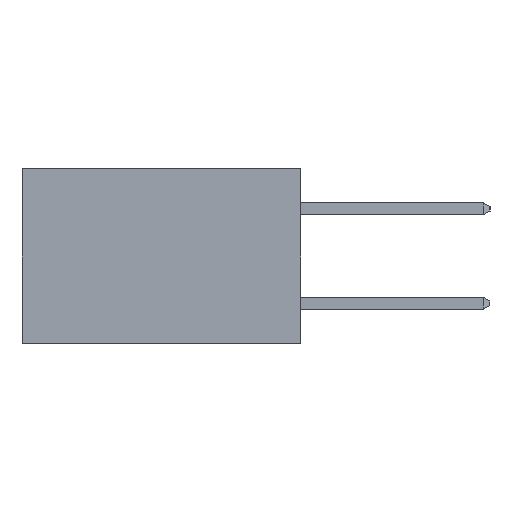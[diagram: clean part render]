
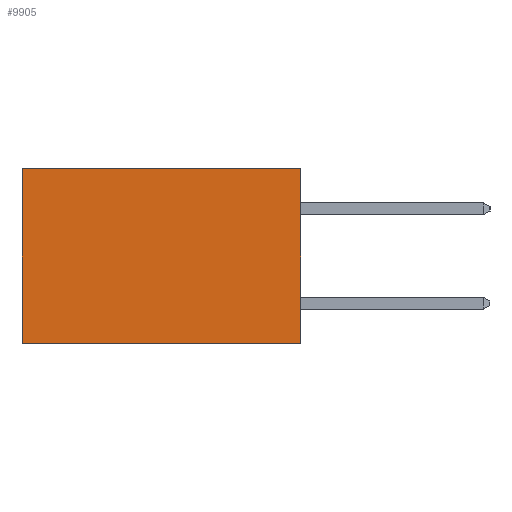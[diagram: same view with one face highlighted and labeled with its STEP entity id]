
A CAD part, left-side view. The second image highlights one B-rep face of the part: STEP entity #9905.
In plain terms, the highlighted planar face has unit normal (-1, 0, 0).
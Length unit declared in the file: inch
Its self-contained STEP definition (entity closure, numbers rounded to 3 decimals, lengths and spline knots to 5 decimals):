
#492 = VECTOR ( 'NONE', #8987, 39.37008 ) ;
#908 = LINE ( 'NONE', #6374, #19864 ) ;
#936 = CARTESIAN_POINT ( 'NONE',  ( 0.277, 0., 0. ) ) ;
#1145 = VERTEX_POINT ( 'NONE', #19620 ) ;
#2804 = DIRECTION ( 'NONE',  ( 1., 0., 0. ) ) ;
#3018 = CARTESIAN_POINT ( 'NONE',  ( 0.277, 0., -0.37 ) ) ;
#3370 = PLANE ( 'NONE',  #23247 ) ;
#4518 = CARTESIAN_POINT ( 'NONE',  ( 0.277, 0., -0.37 ) ) ;
#4908 = EDGE_CURVE ( 'NONE', #19565, #1145, #8633, .T. ) ;
#6332 = DIRECTION ( 'NONE',  ( 0., 0., -1. ) ) ;
#6374 = CARTESIAN_POINT ( 'NONE',  ( 0.277, 0.59, -0.37 ) ) ;
#7234 = VERTEX_POINT ( 'NONE', #936 ) ;
#8633 = LINE ( 'NONE', #8773, #492 ) ;
#8773 = CARTESIAN_POINT ( 'NONE',  ( 0.277, 0., -0.37 ) ) ;
#8987 = DIRECTION ( 'NONE',  ( 0., 1., 0. ) ) ;
#9730 = DIRECTION ( 'NONE',  ( 0., 0., -1. ) ) ;
#9797 = VECTOR ( 'NONE', #19102, 39.37008 ) ;
#9905 = ADVANCED_FACE ( 'NONE', ( #27159 ), #3370, .F. ) ;
#10337 = EDGE_CURVE ( 'NONE', #25428, #1145, #908, .T. ) ;
#13412 = ORIENTED_EDGE ( 'NONE', *, *, #24149, .F. ) ;
#13765 = VECTOR ( 'NONE', #28996, 39.37008 ) ;
#16337 = EDGE_LOOP ( 'NONE', ( #24290, #28705, #13412, #19869 ) ) ;
#16617 = CARTESIAN_POINT ( 'NONE',  ( 0.277, 0., 0. ) ) ;
#19102 = DIRECTION ( 'NONE',  ( 0., 1., 0. ) ) ;
#19565 = VERTEX_POINT ( 'NONE', #29447 ) ;
#19620 = CARTESIAN_POINT ( 'NONE',  ( 0.277, 0.59, -0.37 ) ) ;
#19864 = VECTOR ( 'NONE', #6332, 39.37008 ) ;
#19869 = ORIENTED_EDGE ( 'NONE', *, *, #20085, .T. ) ;
#20085 = EDGE_CURVE ( 'NONE', #7234, #25428, #22854, .T. ) ;
#20301 = LINE ( 'NONE', #4518, #13765 ) ;
#21791 = CARTESIAN_POINT ( 'NONE',  ( 0.277, 0.59, 0. ) ) ;
#22854 = LINE ( 'NONE', #16617, #9797 ) ;
#23247 = AXIS2_PLACEMENT_3D ( 'NONE', #3018, #2804, #9730 ) ;
#24149 = EDGE_CURVE ( 'NONE', #7234, #19565, #20301, .T. ) ;
#24290 = ORIENTED_EDGE ( 'NONE', *, *, #10337, .T. ) ;
#25428 = VERTEX_POINT ( 'NONE', #21791 ) ;
#27159 = FACE_OUTER_BOUND ( 'NONE', #16337, .T. ) ;
#28705 = ORIENTED_EDGE ( 'NONE', *, *, #4908, .F. ) ;
#28996 = DIRECTION ( 'NONE',  ( 0., 0., -1. ) ) ;
#29447 = CARTESIAN_POINT ( 'NONE',  ( 0.277, 0., -0.37 ) ) ;
